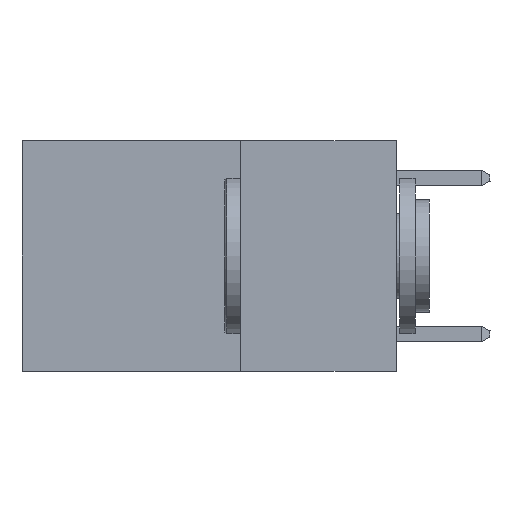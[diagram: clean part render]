
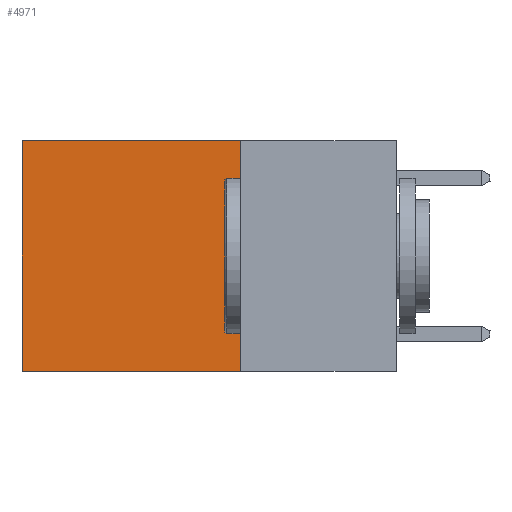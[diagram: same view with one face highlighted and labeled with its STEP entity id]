
A CAD part, left-side view. The second image highlights one B-rep face of the part: STEP entity #4971.
In plain terms, the highlighted planar face has unit normal (-1, 0, 0).
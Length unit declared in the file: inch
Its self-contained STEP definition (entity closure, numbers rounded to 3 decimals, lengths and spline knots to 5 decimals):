
#409 = ORIENTED_EDGE ( 'NONE', *, *, #16758, .F. ) ;
#520 = ORIENTED_EDGE ( 'NONE', *, *, #14069, .T. ) ;
#917 = CARTESIAN_POINT ( 'NONE',  ( 0.2625, 0.6, -0.37 ) ) ;
#996 = EDGE_LOOP ( 'NONE', ( #520, #409, #14618, #27112 ) ) ;
#1151 = LINE ( 'NONE', #21775, #20593 ) ;
#2497 = VERTEX_POINT ( 'NONE', #21796 ) ;
#3871 = DIRECTION ( 'NONE',  ( 1., 0., 0. ) ) ;
#4971 = ADVANCED_FACE ( 'NONE', ( #10168 ), #26622, .F. ) ;
#6620 = CARTESIAN_POINT ( 'NONE',  ( 0.2625, 0.25, -0.37 ) ) ;
#7999 = DIRECTION ( 'NONE',  ( 0., 1., 0. ) ) ;
#8321 = CARTESIAN_POINT ( 'NONE',  ( 0.2625, 0.25, -0.37 ) ) ;
#8375 = VECTOR ( 'NONE', #28079, 39.37008 ) ;
#8621 = DIRECTION ( 'NONE',  ( 0., 1., 0. ) ) ;
#10168 = FACE_OUTER_BOUND ( 'NONE', #996, .T. ) ;
#11029 = LINE ( 'NONE', #8321, #12890 ) ;
#12890 = VECTOR ( 'NONE', #8621, 39.37008 ) ;
#12950 = VECTOR ( 'NONE', #7999, 39.37008 ) ;
#13050 = VERTEX_POINT ( 'NONE', #917 ) ;
#13740 = CARTESIAN_POINT ( 'NONE',  ( 0.2625, 0.25, 0. ) ) ;
#14069 = EDGE_CURVE ( 'NONE', #2497, #13050, #27930, .T. ) ;
#14618 = ORIENTED_EDGE ( 'NONE', *, *, #18424, .F. ) ;
#14716 = CARTESIAN_POINT ( 'NONE',  ( 0.2625, 0.25, 0. ) ) ;
#14865 = LINE ( 'NONE', #14716, #12950 ) ;
#15237 = CARTESIAN_POINT ( 'NONE',  ( 0.2625, 0.25, 0. ) ) ;
#16758 = EDGE_CURVE ( 'NONE', #21020, #13050, #11029, .T. ) ;
#18399 = EDGE_CURVE ( 'NONE', #28622, #2497, #14865, .T. ) ;
#18424 = EDGE_CURVE ( 'NONE', #28622, #21020, #1151, .T. ) ;
#18927 = CARTESIAN_POINT ( 'NONE',  ( 0.2625, 0.6, 0. ) ) ;
#20593 = VECTOR ( 'NONE', #21480, 39.37008 ) ;
#21020 = VERTEX_POINT ( 'NONE', #6620 ) ;
#21480 = DIRECTION ( 'NONE',  ( 0., 0., -1. ) ) ;
#21775 = CARTESIAN_POINT ( 'NONE',  ( 0.2625, 0.25, 0. ) ) ;
#21796 = CARTESIAN_POINT ( 'NONE',  ( 0.2625, 0.6, 0. ) ) ;
#26622 = PLANE ( 'NONE',  #27037 ) ;
#27037 = AXIS2_PLACEMENT_3D ( 'NONE', #15237, #3871, #28444 ) ;
#27112 = ORIENTED_EDGE ( 'NONE', *, *, #18399, .T. ) ;
#27930 = LINE ( 'NONE', #18927, #8375 ) ;
#28079 = DIRECTION ( 'NONE',  ( 0., 0., -1. ) ) ;
#28444 = DIRECTION ( 'NONE',  ( 0., 0., -1. ) ) ;
#28622 = VERTEX_POINT ( 'NONE', #13740 ) ;
